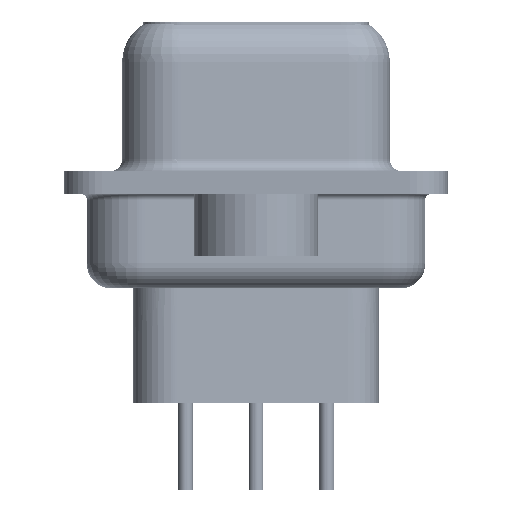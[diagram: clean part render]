
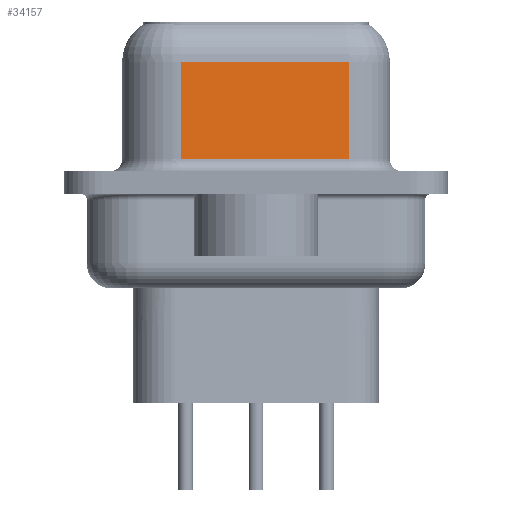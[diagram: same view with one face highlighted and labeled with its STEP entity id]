
A CAD part, left-side view. The second image highlights one B-rep face of the part: STEP entity #34157.
In plain terms, the highlighted planar face has unit normal (-0.985, -0.174, 0).
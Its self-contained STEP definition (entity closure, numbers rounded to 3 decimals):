
#396 = VECTOR ( 'NONE', #19322, 1000. ) ;
#4211 = CARTESIAN_POINT ( 'NONE',  ( 4.43, 3.028, 0.95 ) ) ;
#5864 = VERTEX_POINT ( 'NONE', #4211 ) ;
#8720 = ORIENTED_EDGE ( 'NONE', *, *, #42712, .T. ) ;
#8986 = CARTESIAN_POINT ( 'NONE',  ( 4.43, 3.028, 4.85 ) ) ;
#9815 = ORIENTED_EDGE ( 'NONE', *, *, #34828, .T. ) ;
#9861 = VERTEX_POINT ( 'NONE', #34686 ) ;
#9912 = DIRECTION ( 'NONE',  ( -0.174, 0.985, 0. ) ) ;
#11643 = DIRECTION ( 'NONE',  ( 0.985, 0.174, 0. ) ) ;
#13087 = LINE ( 'NONE', #20347, #38939 ) ;
#15028 = VECTOR ( 'NONE', #9912, 1000. ) ;
#16973 = LINE ( 'NONE', #31246, #15028 ) ;
#16996 = EDGE_LOOP ( 'NONE', ( #28201, #9815, #8720, #36115 ) ) ;
#17685 = EDGE_CURVE ( 'NONE', #5864, #9861, #33385, .T. ) ;
#19043 = VECTOR ( 'NONE', #30344, 1000. ) ;
#19322 = DIRECTION ( 'NONE',  ( 0., 0., -1. ) ) ;
#19617 = DIRECTION ( 'NONE',  ( -0.174, 0.985, 0. ) ) ;
#20107 = DIRECTION ( 'NONE',  ( 0., 0., -1. ) ) ;
#20347 = CARTESIAN_POINT ( 'NONE',  ( 5.621, -3.722, 6.6 ) ) ;
#20874 = AXIS2_PLACEMENT_3D ( 'NONE', #36921, #11643, #19617 ) ;
#21390 = VERTEX_POINT ( 'NONE', #8986 ) ;
#22671 = FACE_OUTER_BOUND ( 'NONE', #16996, .T. ) ;
#28201 = ORIENTED_EDGE ( 'NONE', *, *, #36775, .F. ) ;
#30344 = DIRECTION ( 'NONE',  ( 0.174, -0.985, 0. ) ) ;
#30379 = PLANE ( 'NONE',  #20874 ) ;
#31246 = CARTESIAN_POINT ( 'NONE',  ( 5.621, -3.722, 4.85 ) ) ;
#33385 = LINE ( 'NONE', #41323, #19043 ) ;
#34157 = ADVANCED_FACE ( 'NONE', ( #22671 ), #30379, .F. ) ;
#34686 = CARTESIAN_POINT ( 'NONE',  ( 5.621, -3.722, 0.95 ) ) ;
#34828 = EDGE_CURVE ( 'NONE', #36128, #21390, #16973, .T. ) ;
#36115 = ORIENTED_EDGE ( 'NONE', *, *, #17685, .T. ) ;
#36128 = VERTEX_POINT ( 'NONE', #38919 ) ;
#36775 = EDGE_CURVE ( 'NONE', #36128, #9861, #13087, .T. ) ;
#36921 = CARTESIAN_POINT ( 'NONE',  ( 5.621, -3.722, 6.6 ) ) ;
#37791 = LINE ( 'NONE', #44611, #396 ) ;
#38919 = CARTESIAN_POINT ( 'NONE',  ( 5.621, -3.722, 4.85 ) ) ;
#38939 = VECTOR ( 'NONE', #20107, 1000. ) ;
#41323 = CARTESIAN_POINT ( 'NONE',  ( 5.621, -3.722, 0.95 ) ) ;
#42712 = EDGE_CURVE ( 'NONE', #21390, #5864, #37791, .T. ) ;
#44611 = CARTESIAN_POINT ( 'NONE',  ( 4.43, 3.028, 6.6 ) ) ;
